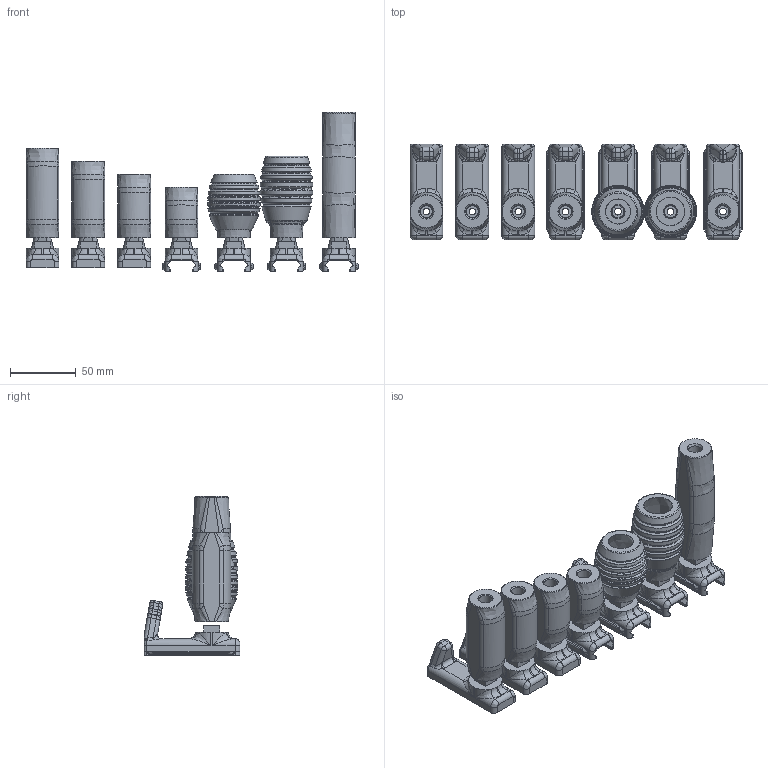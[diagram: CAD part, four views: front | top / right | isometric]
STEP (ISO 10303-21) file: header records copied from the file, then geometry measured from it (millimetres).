
FILE_DESCRIPTION(/* description */ (''),/* implementation_level */ '2;1');
FILE_NAME(/* name */ 'MOD GRIP V5.stp',/* time_stamp */ '2020-04-12T12:29:01+03:00',/* author */ (''),/* organization */ (''),/* preprocessor_version */ 'ST-DEVELOPER v15.2',/* originating_system */ 'Autodesk Translator Framework v2.0.0.5431',/* authorisation */ '');
FILE_SCHEMA (('AUTOMOTIVE_DESIGN { 1 0 10303 214 3 1 1 }'));
Products named in the file (1): MOD GRIP V5
Bounding box: 253 x 73.03 x 121.65 mm (x, y, z)
Volume: 368388.1 mm3; surface area: 122033.2 mm2
Topology: 14 solids, 14 shells, 1476 faces, 3482 edges, 2053 vertices
Faces by surface type: bspline 549, plane 413, cylinder 384, cone 55, torus 49, sphere 26
Full cylindrical faces by diameter (mm): 4 x6, 5 x5, 5.2 x2, 5.5 x4, 6 x3, 10 x7
Entity records: 60604 total; most frequent: CARTESIAN_POINT 29507, ORIENTED_EDGE 6806, DIRECTION 5697, EDGE_CURVE 3403, AXIS2_PLACEMENT_3D 2178, VERTEX_POINT 2050, EDGE_LOOP 1599, ADVANCED_FACE 1476
